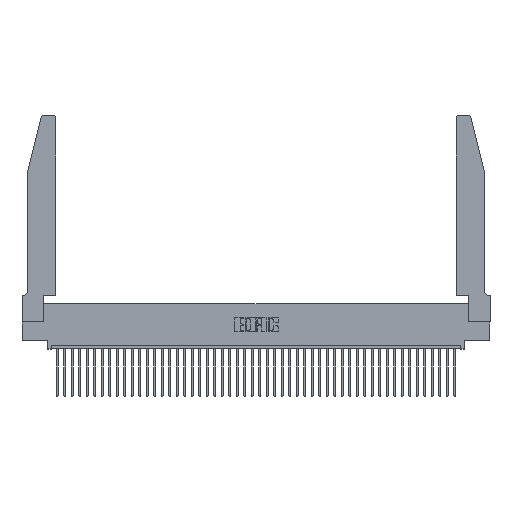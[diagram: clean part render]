
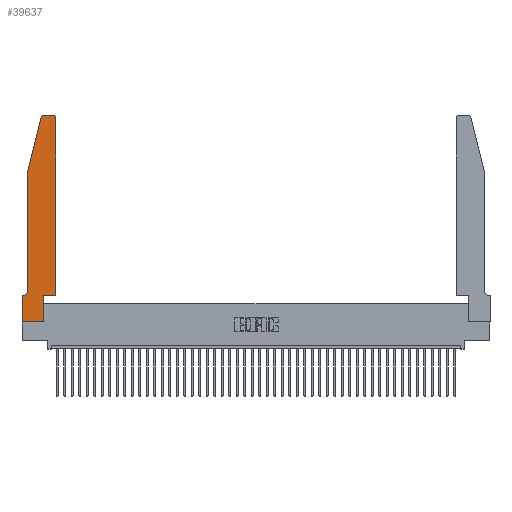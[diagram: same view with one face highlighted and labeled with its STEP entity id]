
A CAD part, top view. The second image highlights one B-rep face of the part: STEP entity #39637.
In plain terms, the highlighted planar face has unit normal (0, 0, 1).
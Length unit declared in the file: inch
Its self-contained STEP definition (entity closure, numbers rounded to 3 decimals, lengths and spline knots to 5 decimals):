
#532 = ORIENTED_EDGE ( 'NONE', *, *, #38897, .T. ) ;
#643 = LINE ( 'NONE', #1917, #33160 ) ;
#1820 = ORIENTED_EDGE ( 'NONE', *, *, #11907, .T. ) ;
#1917 = CARTESIAN_POINT ( 'NONE',  ( 0.0755, 2., 0.37 ) ) ;
#1926 = EDGE_CURVE ( 'NONE', #41202, #12761, #30578, .T. ) ;
#2147 = CARTESIAN_POINT ( 'NONE',  ( 0.0055, 0.35, 0.37 ) ) ;
#2353 = CARTESIAN_POINT ( 'NONE',  ( 0., 0., 0.37 ) ) ;
#3027 = VERTEX_POINT ( 'NONE', #8464 ) ;
#3520 = CARTESIAN_POINT ( 'NONE',  ( 0.0755, 2., 0.37 ) ) ;
#3632 = DIRECTION ( 'NONE',  ( 0., -1., 0. ) ) ;
#3650 = ORIENTED_EDGE ( 'NONE', *, *, #33380, .T. ) ;
#3954 = LINE ( 'NONE', #36554, #41080 ) ;
#3990 = DIRECTION ( 'NONE',  ( 1., 0., 0. ) ) ;
#4613 = CARTESIAN_POINT ( 'NONE',  ( 0.2865, 0.35, 0.37 ) ) ;
#5058 = VERTEX_POINT ( 'NONE', #16199 ) ;
#5717 = ORIENTED_EDGE ( 'NONE', *, *, #35268, .T. ) ;
#6009 = DIRECTION ( 'NONE',  ( 0., 1., 0. ) ) ;
#6760 = LINE ( 'NONE', #12974, #24323 ) ;
#6949 = FACE_OUTER_BOUND ( 'NONE', #33169, .T. ) ;
#8355 = LINE ( 'NONE', #24115, #33374 ) ;
#8464 = CARTESIAN_POINT ( 'NONE',  ( 0.284, 2.75, 0.37 ) ) ;
#8789 = VERTEX_POINT ( 'NONE', #3520 ) ;
#9949 = PLANE ( 'NONE',  #32066 ) ;
#9952 = ORIENTED_EDGE ( 'NONE', *, *, #10522, .T. ) ;
#10522 = EDGE_CURVE ( 'NONE', #35990, #34210, #11958, .T. ) ;
#10968 = LINE ( 'NONE', #13960, #34391 ) ;
#11907 = EDGE_CURVE ( 'NONE', #5058, #8789, #643, .T. ) ;
#11958 = CIRCLE ( 'NONE', #19621, 0.03 ) ;
#12761 = VERTEX_POINT ( 'NONE', #2147 ) ;
#12974 = CARTESIAN_POINT ( 'NONE',  ( 0.2605, 2.75, 0.37 ) ) ;
#13061 = CARTESIAN_POINT ( 'NONE',  ( 0., 0., 0.37 ) ) ;
#13960 = CARTESIAN_POINT ( 'NONE',  ( 0.0755, 2., 0.37 ) ) ;
#14732 = VERTEX_POINT ( 'NONE', #22815 ) ;
#14740 = DIRECTION ( 'NONE',  ( 1., 0., 0. ) ) ;
#14904 = CARTESIAN_POINT ( 'NONE',  ( 0., 0., 0.37 ) ) ;
#14920 = ORIENTED_EDGE ( 'NONE', *, *, #1926, .T. ) ;
#14950 = VECTOR ( 'NONE', #6009, 39.37008 ) ;
#15282 = ORIENTED_EDGE ( 'NONE', *, *, #33761, .T. ) ;
#15329 = AXIS2_PLACEMENT_3D ( 'NONE', #22749, #26150, #43159 ) ;
#15719 = LINE ( 'NONE', #14904, #42754 ) ;
#16199 = CARTESIAN_POINT ( 'NONE',  ( 0.25487, 2.72718, 0.37 ) ) ;
#16362 = CARTESIAN_POINT ( 'NONE',  ( 0.4505, 0.35, 0.37 ) ) ;
#17468 = DIRECTION ( 'NONE',  ( 0., 0., 1. ) ) ;
#17724 = DIRECTION ( 'NONE',  ( -0.239, -0.971, 0. ) ) ;
#17871 = CARTESIAN_POINT ( 'NONE',  ( 0.4505, 0.35, 0.37 ) ) ;
#18741 = VECTOR ( 'NONE', #14740, 39.37008 ) ;
#19603 = DIRECTION ( 'NONE',  ( 1., 0., 0. ) ) ;
#19621 = AXIS2_PLACEMENT_3D ( 'NONE', #21785, #29091, #42350 ) ;
#19806 = DIRECTION ( 'NONE',  ( -1., 0., 0. ) ) ;
#20703 = VERTEX_POINT ( 'NONE', #35045 ) ;
#21785 = CARTESIAN_POINT ( 'NONE',  ( 0.4205, 2.72, 0.37 ) ) ;
#22469 = LINE ( 'NONE', #17871, #18741 ) ;
#22749 = CARTESIAN_POINT ( 'NONE',  ( 0.0055, 0.42, 0.37 ) ) ;
#22815 = CARTESIAN_POINT ( 'NONE',  ( 0., 0.35, 0.37 ) ) ;
#23002 = ORIENTED_EDGE ( 'NONE', *, *, #41527, .T. ) ;
#24115 = CARTESIAN_POINT ( 'NONE',  ( 0.2865, 0.35, 0.37 ) ) ;
#24323 = VECTOR ( 'NONE', #19806, 39.37008 ) ;
#24499 = CARTESIAN_POINT ( 'NONE',  ( 0.284, 2.72, 0.37 ) ) ;
#24921 = VERTEX_POINT ( 'NONE', #42453 ) ;
#24928 = EDGE_CURVE ( 'NONE', #12761, #14732, #3954, .T. ) ;
#24983 = CARTESIAN_POINT ( 'NONE',  ( 0.4505, 2.72, 0.37 ) ) ;
#25239 = EDGE_CURVE ( 'NONE', #3027, #5058, #35885, .T. ) ;
#25458 = ORIENTED_EDGE ( 'NONE', *, *, #41621, .T. ) ;
#25915 = AXIS2_PLACEMENT_3D ( 'NONE', #24499, #17468, #3990 ) ;
#26150 = DIRECTION ( 'NONE',  ( 0., 0., -1. ) ) ;
#29091 = DIRECTION ( 'NONE',  ( 0., 0., 1. ) ) ;
#29242 = VERTEX_POINT ( 'NONE', #2353 ) ;
#30290 = ORIENTED_EDGE ( 'NONE', *, *, #41696, .T. ) ;
#30578 = CIRCLE ( 'NONE', #15329, 0.07 ) ;
#31377 = ORIENTED_EDGE ( 'NONE', *, *, #24928, .T. ) ;
#31457 = VERTEX_POINT ( 'NONE', #4613 ) ;
#31583 = DIRECTION ( 'NONE',  ( -1., 0., 0. ) ) ;
#32066 = AXIS2_PLACEMENT_3D ( 'NONE', #36816, #36515, #37118 ) ;
#32394 = ORIENTED_EDGE ( 'NONE', *, *, #25239, .T. ) ;
#33160 = VECTOR ( 'NONE', #17724, 39.37008 ) ;
#33169 = EDGE_LOOP ( 'NONE', ( #23002, #32394, #1820, #30290, #14920, #31377, #15282, #3650, #25458, #5717, #532, #9952 ) ) ;
#33343 = VECTOR ( 'NONE', #19603, 39.37008 ) ;
#33374 = VECTOR ( 'NONE', #37601, 39.37008 ) ;
#33380 = EDGE_CURVE ( 'NONE', #29242, #20703, #38573, .T. ) ;
#33761 = EDGE_CURVE ( 'NONE', #14732, #29242, #15719, .T. ) ;
#34210 = VERTEX_POINT ( 'NONE', #34634 ) ;
#34391 = VECTOR ( 'NONE', #3632, 39.37008 ) ;
#34634 = CARTESIAN_POINT ( 'NONE',  ( 0.4205, 2.75, 0.37 ) ) ;
#35045 = CARTESIAN_POINT ( 'NONE',  ( 0.2865, 0., 0.37 ) ) ;
#35268 = EDGE_CURVE ( 'NONE', #31457, #24921, #22469, .T. ) ;
#35885 = CIRCLE ( 'NONE', #25915, 0.03 ) ;
#35990 = VERTEX_POINT ( 'NONE', #24983 ) ;
#36515 = DIRECTION ( 'NONE',  ( 0., 0., 1. ) ) ;
#36554 = CARTESIAN_POINT ( 'NONE',  ( 0.0755, 0.35, 0.37 ) ) ;
#36816 = CARTESIAN_POINT ( 'NONE',  ( 0., 0.35, 0.37 ) ) ;
#37118 = DIRECTION ( 'NONE',  ( 1., 0., 0. ) ) ;
#37601 = DIRECTION ( 'NONE',  ( 0., 1., 0. ) ) ;
#38573 = LINE ( 'NONE', #13061, #33343 ) ;
#38897 = EDGE_CURVE ( 'NONE', #24921, #35990, #43090, .T. ) ;
#38952 = DIRECTION ( 'NONE',  ( 0., -1., 0. ) ) ;
#39637 = ADVANCED_FACE ( 'NONE', ( #6949 ), #9949, .T. ) ;
#41080 = VECTOR ( 'NONE', #31583, 39.37008 ) ;
#41202 = VERTEX_POINT ( 'NONE', #41852 ) ;
#41527 = EDGE_CURVE ( 'NONE', #34210, #3027, #6760, .T. ) ;
#41621 = EDGE_CURVE ( 'NONE', #20703, #31457, #8355, .T. ) ;
#41696 = EDGE_CURVE ( 'NONE', #8789, #41202, #10968, .T. ) ;
#41852 = CARTESIAN_POINT ( 'NONE',  ( 0.0755, 0.42, 0.37 ) ) ;
#42350 = DIRECTION ( 'NONE',  ( 1., 0., 0. ) ) ;
#42453 = CARTESIAN_POINT ( 'NONE',  ( 0.4505, 0.35, 0.37 ) ) ;
#42754 = VECTOR ( 'NONE', #38952, 39.37008 ) ;
#43090 = LINE ( 'NONE', #16362, #14950 ) ;
#43159 = DIRECTION ( 'NONE',  ( -1., 0., 0. ) ) ;
